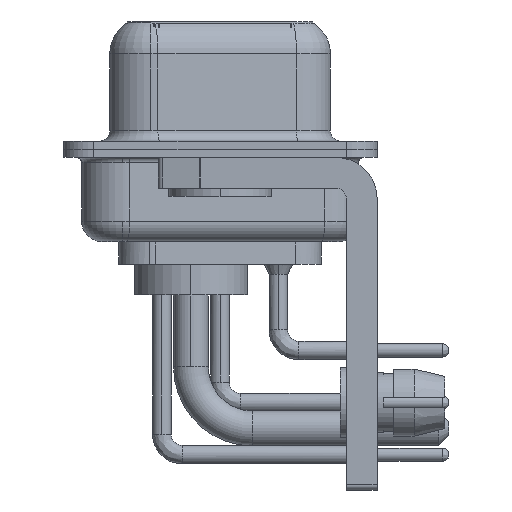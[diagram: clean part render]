
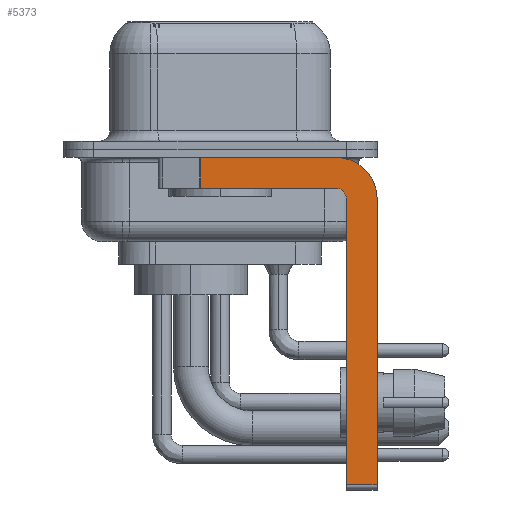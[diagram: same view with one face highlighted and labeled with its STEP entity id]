
A CAD part, left-side view. The second image highlights one B-rep face of the part: STEP entity #5373.
In plain terms, the highlighted planar face has unit normal (-1, 0, 0).
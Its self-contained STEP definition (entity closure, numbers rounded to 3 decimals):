
#756 = VECTOR ( 'NONE', #3411, 1000. ) ;
#1321 = CARTESIAN_POINT ( 'NONE',  ( -2.9, -5.65, -2.4 ) ) ;
#2898 = LINE ( 'NONE', #13653, #756 ) ;
#3411 = DIRECTION ( 'NONE',  ( 0., -1., 0. ) ) ;
#4262 = EDGE_CURVE ( 'NONE', #29934, #34894, #2898, .T. ) ;
#4360 = ORIENTED_EDGE ( 'NONE', *, *, #27274, .T. ) ;
#4626 = AXIS2_PLACEMENT_3D ( 'NONE', #1321, #7340, #23013 ) ;
#5194 = LINE ( 'NONE', #15924, #13870 ) ;
#5373 = ADVANCED_FACE ( 'NONE', ( #25861 ), #9990, .F. ) ;
#5422 = DIRECTION ( 'NONE',  ( 0., -1., 0. ) ) ;
#7340 = DIRECTION ( 'NONE',  ( 1., 0., 0. ) ) ;
#7421 = VERTEX_POINT ( 'NONE', #8421 ) ;
#8421 = CARTESIAN_POINT ( 'NONE',  ( -2.9, 0.978, -1.9 ) ) ;
#9341 = CARTESIAN_POINT ( 'NONE',  ( -2.9, -6.15, -16.35 ) ) ;
#9546 = ORIENTED_EDGE ( 'NONE', *, *, #25386, .F. ) ;
#9552 = CARTESIAN_POINT ( 'NONE',  ( -2.9, -7.65, -2.4 ) ) ;
#9724 = ORIENTED_EDGE ( 'NONE', *, *, #20159, .F. ) ;
#9990 = PLANE ( 'NONE',  #4626 ) ;
#10386 = EDGE_CURVE ( 'NONE', #15897, #33896, #31664, .T. ) ;
#11443 = AXIS2_PLACEMENT_3D ( 'NONE', #25691, #23211, #25336 ) ;
#12622 = DIRECTION ( 'NONE',  ( -1., 0., 0. ) ) ;
#12783 = DIRECTION ( 'NONE',  ( 0., 0., -1. ) ) ;
#13347 = LINE ( 'NONE', #18449, #29951 ) ;
#13653 = CARTESIAN_POINT ( 'NONE',  ( -2.9, 3., -0.4 ) ) ;
#13870 = VECTOR ( 'NONE', #12783, 1000. ) ;
#14071 = CARTESIAN_POINT ( 'NONE',  ( -2.9, 0.978, -0.4 ) ) ;
#15244 = CARTESIAN_POINT ( 'NONE',  ( -2.9, -5.65, -2.4 ) ) ;
#15897 = VERTEX_POINT ( 'NONE', #20524 ) ;
#15924 = CARTESIAN_POINT ( 'NONE',  ( -2.9, 0.978, -1.9 ) ) ;
#17524 = VERTEX_POINT ( 'NONE', #9552 ) ;
#17564 = EDGE_CURVE ( 'NONE', #33896, #7421, #28435, .T. ) ;
#17596 = VERTEX_POINT ( 'NONE', #28247 ) ;
#18449 = CARTESIAN_POINT ( 'NONE',  ( -2.9, -5.65, -16.35 ) ) ;
#18713 = VECTOR ( 'NONE', #32942, 1000. ) ;
#19984 = ORIENTED_EDGE ( 'NONE', *, *, #34508, .T. ) ;
#20159 = EDGE_CURVE ( 'NONE', #17524, #17596, #27343, .T. ) ;
#20453 = CARTESIAN_POINT ( 'NONE',  ( -2.9, -5.65, -1.9 ) ) ;
#20524 = CARTESIAN_POINT ( 'NONE',  ( -2.9, -6.15, -2.4 ) ) ;
#20701 = DIRECTION ( 'NONE',  ( 0., 0., 1. ) ) ;
#21304 = ORIENTED_EDGE ( 'NONE', *, *, #25241, .F. ) ;
#21491 = AXIS2_PLACEMENT_3D ( 'NONE', #15244, #12622, #20701 ) ;
#22392 = ORIENTED_EDGE ( 'NONE', *, *, #10386, .F. ) ;
#23013 = DIRECTION ( 'NONE',  ( 0., 0., -1. ) ) ;
#23211 = DIRECTION ( 'NONE',  ( 1., 0., 0. ) ) ;
#23276 = ORIENTED_EDGE ( 'NONE', *, *, #4262, .F. ) ;
#23535 = CARTESIAN_POINT ( 'NONE',  ( -2.9, -5.65, -0.4 ) ) ;
#24363 = CIRCLE ( 'NONE', #11443, 2. ) ;
#24458 = CARTESIAN_POINT ( 'NONE',  ( -2.9, -6.15, -16.6 ) ) ;
#25241 = EDGE_CURVE ( 'NONE', #31554, #15897, #33111, .T. ) ;
#25336 = DIRECTION ( 'NONE',  ( 0., 0., -1. ) ) ;
#25386 = EDGE_CURVE ( 'NONE', #34894, #17524, #24363, .T. ) ;
#25691 = CARTESIAN_POINT ( 'NONE',  ( -2.9, -5.65, -2.4 ) ) ;
#25861 = FACE_OUTER_BOUND ( 'NONE', #32287, .T. ) ;
#27274 = EDGE_CURVE ( 'NONE', #29934, #7421, #5194, .T. ) ;
#27343 = LINE ( 'NONE', #30171, #33121 ) ;
#28247 = CARTESIAN_POINT ( 'NONE',  ( -2.9, -7.65, -16.35 ) ) ;
#28435 = LINE ( 'NONE', #20453, #31966 ) ;
#28963 = CARTESIAN_POINT ( 'NONE',  ( -2.9, -5.65, -1.9 ) ) ;
#29934 = VERTEX_POINT ( 'NONE', #14071 ) ;
#29951 = VECTOR ( 'NONE', #5422, 1000. ) ;
#30171 = CARTESIAN_POINT ( 'NONE',  ( -2.9, -7.65, -2.4 ) ) ;
#30899 = DIRECTION ( 'NONE',  ( 0., 1., 0. ) ) ;
#31554 = VERTEX_POINT ( 'NONE', #9341 ) ;
#31664 = CIRCLE ( 'NONE', #21491, 0.5 ) ;
#31699 = ORIENTED_EDGE ( 'NONE', *, *, #17564, .F. ) ;
#31966 = VECTOR ( 'NONE', #30899, 1000. ) ;
#32287 = EDGE_LOOP ( 'NONE', ( #23276, #4360, #31699, #22392, #21304, #19984, #9724, #9546 ) ) ;
#32480 = DIRECTION ( 'NONE',  ( 0., 0., -1. ) ) ;
#32942 = DIRECTION ( 'NONE',  ( 0., 0., 1. ) ) ;
#33111 = LINE ( 'NONE', #24458, #18713 ) ;
#33121 = VECTOR ( 'NONE', #32480, 1000. ) ;
#33896 = VERTEX_POINT ( 'NONE', #28963 ) ;
#34508 = EDGE_CURVE ( 'NONE', #31554, #17596, #13347, .T. ) ;
#34894 = VERTEX_POINT ( 'NONE', #23535 ) ;
